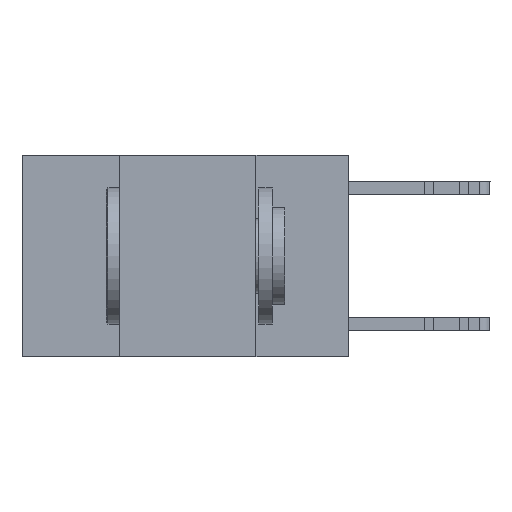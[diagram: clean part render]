
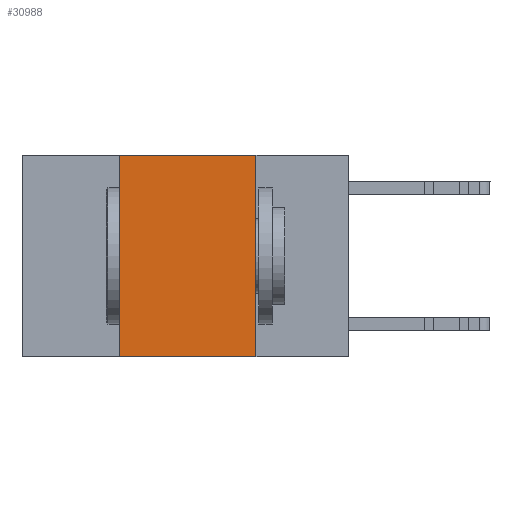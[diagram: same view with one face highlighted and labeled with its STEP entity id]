
A CAD part, left-side view. The second image highlights one B-rep face of the part: STEP entity #30988.
In plain terms, the highlighted planar face has unit normal (-1, 0, 0).
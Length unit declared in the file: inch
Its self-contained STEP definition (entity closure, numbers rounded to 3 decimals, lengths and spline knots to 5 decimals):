
#419 = DIRECTION ( 'NONE',  ( 0., -1., 0. ) ) ;
#421 = ORIENTED_EDGE ( 'NONE', *, *, #18397, .T. ) ;
#447 = VERTEX_POINT ( 'NONE', #6203 ) ;
#748 = AXIS2_PLACEMENT_3D ( 'NONE', #9789, #15095, #10118 ) ;
#2721 = VECTOR ( 'NONE', #25800, 39.37008 ) ;
#2826 = VERTEX_POINT ( 'NONE', #29172 ) ;
#3959 = DIRECTION ( 'NONE',  ( 0., 0., -1. ) ) ;
#4276 = VECTOR ( 'NONE', #419, 39.37008 ) ;
#4688 = ORIENTED_EDGE ( 'NONE', *, *, #18213, .F. ) ;
#6046 = ORIENTED_EDGE ( 'NONE', *, *, #10156, .F. ) ;
#6092 = LINE ( 'NONE', #8251, #2721 ) ;
#6203 = CARTESIAN_POINT ( 'NONE',  ( 0., 0.17, 0. ) ) ;
#6569 = LINE ( 'NONE', #22285, #16500 ) ;
#6798 = ORIENTED_EDGE ( 'NONE', *, *, #22988, .F. ) ;
#7086 = VECTOR ( 'NONE', #3959, 39.37008 ) ;
#8251 = CARTESIAN_POINT ( 'NONE',  ( 0., 0.42, 0. ) ) ;
#8652 = EDGE_LOOP ( 'NONE', ( #6798, #6046, #4688, #421 ) ) ;
#9445 = FACE_OUTER_BOUND ( 'NONE', #8652, .T. ) ;
#9472 = CARTESIAN_POINT ( 'NONE',  ( 0., 0.17, -0.37 ) ) ;
#9789 = CARTESIAN_POINT ( 'NONE',  ( 0., 0.6, 0. ) ) ;
#10118 = DIRECTION ( 'NONE',  ( 0., 0., -1. ) ) ;
#10156 = EDGE_CURVE ( 'NONE', #2826, #447, #25428, .T. ) ;
#13018 = CARTESIAN_POINT ( 'NONE',  ( 0., 0.6, 0. ) ) ;
#13392 = VERTEX_POINT ( 'NONE', #9472 ) ;
#13768 = VERTEX_POINT ( 'NONE', #14089 ) ;
#14044 = DIRECTION ( 'NONE',  ( 0., -1., 0. ) ) ;
#14089 = CARTESIAN_POINT ( 'NONE',  ( 0., 0.42, -0.37 ) ) ;
#15095 = DIRECTION ( 'NONE',  ( 1., 0., 0. ) ) ;
#16500 = VECTOR ( 'NONE', #14044, 39.37008 ) ;
#18213 = EDGE_CURVE ( 'NONE', #13768, #2826, #6092, .T. ) ;
#18397 = EDGE_CURVE ( 'NONE', #13768, #13392, #6569, .T. ) ;
#22285 = CARTESIAN_POINT ( 'NONE',  ( 0., 0.6, -0.37 ) ) ;
#22988 = EDGE_CURVE ( 'NONE', #447, #13392, #29150, .T. ) ;
#25428 = LINE ( 'NONE', #13018, #4276 ) ;
#25800 = DIRECTION ( 'NONE',  ( 0., 0., 1. ) ) ;
#26801 = CARTESIAN_POINT ( 'NONE',  ( 0., 0.17, 0. ) ) ;
#29150 = LINE ( 'NONE', #26801, #7086 ) ;
#29172 = CARTESIAN_POINT ( 'NONE',  ( 0., 0.42, 0. ) ) ;
#30988 = ADVANCED_FACE ( 'NONE', ( #9445 ), #32494, .F. ) ;
#32494 = PLANE ( 'NONE',  #748 ) ;
